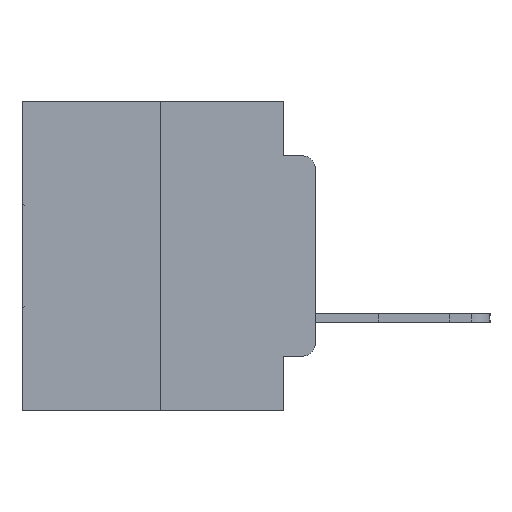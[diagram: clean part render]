
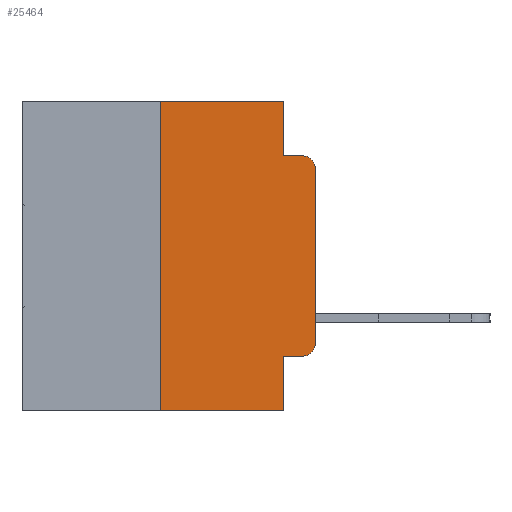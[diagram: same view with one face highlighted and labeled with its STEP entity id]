
A CAD part, left-side view. The second image highlights one B-rep face of the part: STEP entity #25464.
In plain terms, the highlighted planar face has unit normal (-1, 0, 0).
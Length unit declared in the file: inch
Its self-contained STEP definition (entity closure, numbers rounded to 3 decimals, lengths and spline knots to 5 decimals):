
#554 = AXIS2_PLACEMENT_3D ( 'NONE', #18493, #17868, #17990 ) ;
#778 = CARTESIAN_POINT ( 'NONE',  ( 0., 0., -0.1085 ) ) ;
#1525 = EDGE_CURVE ( 'NONE', #25585, #26327, #14648, .T. ) ;
#2395 = ORIENTED_EDGE ( 'NONE', *, *, #7699, .F. ) ;
#3117 = EDGE_CURVE ( 'NONE', #27925, #25585, #3892, .T. ) ;
#3740 = LINE ( 'NONE', #4854, #8344 ) ;
#3865 = DIRECTION ( 'NONE',  ( 0., 0., -1. ) ) ;
#3892 = LINE ( 'NONE', #23694, #26974 ) ;
#4602 = CARTESIAN_POINT ( 'NONE',  ( 0., 0.051, 0. ) ) ;
#4655 = LINE ( 'NONE', #24834, #6081 ) ;
#4662 = EDGE_CURVE ( 'NONE', #27925, #23006, #21340, .T. ) ;
#4854 = CARTESIAN_POINT ( 'NONE',  ( 0., 0.051, -0.0885 ) ) ;
#5065 = VECTOR ( 'NONE', #11693, 39.37008 ) ;
#5301 = CARTESIAN_POINT ( 'NONE',  ( 0., 0.02, -0.0885 ) ) ;
#5423 = ORIENTED_EDGE ( 'NONE', *, *, #21184, .T. ) ;
#6081 = VECTOR ( 'NONE', #16053, 39.37008 ) ;
#6410 = EDGE_CURVE ( 'NONE', #25180, #23006, #28482, .T. ) ;
#7229 = CARTESIAN_POINT ( 'NONE',  ( 0., 0.051, 0. ) ) ;
#7239 = VERTEX_POINT ( 'NONE', #778 ) ;
#7511 = ORIENTED_EDGE ( 'NONE', *, *, #3117, .T. ) ;
#7691 = VECTOR ( 'NONE', #21485, 39.37008 ) ;
#7699 = EDGE_CURVE ( 'NONE', #25180, #12014, #11096, .T. ) ;
#8344 = VECTOR ( 'NONE', #20522, 39.37008 ) ;
#8591 = ORIENTED_EDGE ( 'NONE', *, *, #1525, .T. ) ;
#8647 = CARTESIAN_POINT ( 'NONE',  ( 0., 0.051, -0.5 ) ) ;
#9223 = EDGE_CURVE ( 'NONE', #25778, #20051, #13744, .T. ) ;
#9306 = CARTESIAN_POINT ( 'NONE',  ( 0., 0.473, 0. ) ) ;
#9703 = ORIENTED_EDGE ( 'NONE', *, *, #10740, .F. ) ;
#10339 = DIRECTION ( 'NONE',  ( 0., -1., 0. ) ) ;
#10424 = VECTOR ( 'NONE', #22671, 39.37008 ) ;
#10740 = EDGE_CURVE ( 'NONE', #20051, #24617, #3740, .T. ) ;
#10778 = VECTOR ( 'NONE', #24405, 39.37008 ) ;
#11096 = LINE ( 'NONE', #18317, #5065 ) ;
#11348 = DIRECTION ( 'NONE',  ( 0., 0., -1. ) ) ;
#11401 = DIRECTION ( 'NONE',  ( -1., 0., 0. ) ) ;
#11693 = DIRECTION ( 'NONE',  ( 0., 0., 1. ) ) ;
#12014 = VERTEX_POINT ( 'NONE', #28065 ) ;
#12243 = CARTESIAN_POINT ( 'NONE',  ( 0., 0.051, -0.0885 ) ) ;
#12631 = CIRCLE ( 'NONE', #14117, 0.02 ) ;
#12891 = PLANE ( 'NONE',  #17390 ) ;
#13077 = ORIENTED_EDGE ( 'NONE', *, *, #18103, .F. ) ;
#13744 = LINE ( 'NONE', #21589, #7691 ) ;
#13746 = CARTESIAN_POINT ( 'NONE',  ( 0., 0., -0.3915 ) ) ;
#14117 = AXIS2_PLACEMENT_3D ( 'NONE', #24721, #11401, #26929 ) ;
#14648 = CIRCLE ( 'NONE', #554, 0.02 ) ;
#15046 = LINE ( 'NONE', #9306, #10424 ) ;
#15090 = CARTESIAN_POINT ( 'NONE',  ( 0., 0.473, 0. ) ) ;
#15502 = VECTOR ( 'NONE', #11348, 39.37008 ) ;
#15559 = CARTESIAN_POINT ( 'NONE',  ( 0., 0.02, -0.4115 ) ) ;
#16053 = DIRECTION ( 'NONE',  ( 0., 0., 1. ) ) ;
#16737 = ORIENTED_EDGE ( 'NONE', *, *, #16756, .T. ) ;
#16756 = EDGE_CURVE ( 'NONE', #7239, #24617, #12631, .T. ) ;
#17208 = ORIENTED_EDGE ( 'NONE', *, *, #9223, .F. ) ;
#17357 = DIRECTION ( 'NONE',  ( 1., 0., 0. ) ) ;
#17390 = AXIS2_PLACEMENT_3D ( 'NONE', #15090, #17357, #3865 ) ;
#17868 = DIRECTION ( 'NONE',  ( -1., 0., 0. ) ) ;
#17990 = DIRECTION ( 'NONE',  ( 0., 0., -1. ) ) ;
#18103 = EDGE_CURVE ( 'NONE', #12014, #25778, #15046, .T. ) ;
#18317 = CARTESIAN_POINT ( 'NONE',  ( 0., 0.25, 0. ) ) ;
#18493 = CARTESIAN_POINT ( 'NONE',  ( 0., 0.02, -0.3915 ) ) ;
#18513 = CARTESIAN_POINT ( 'NONE',  ( 0., 0.25, -0.5 ) ) ;
#19915 = CARTESIAN_POINT ( 'NONE',  ( 0., 0.473, -0.5 ) ) ;
#20051 = VERTEX_POINT ( 'NONE', #12243 ) ;
#20522 = DIRECTION ( 'NONE',  ( 0., -1., 0. ) ) ;
#21152 = FACE_OUTER_BOUND ( 'NONE', #21882, .T. ) ;
#21184 = EDGE_CURVE ( 'NONE', #26327, #7239, #4655, .T. ) ;
#21340 = LINE ( 'NONE', #4602, #15502 ) ;
#21485 = DIRECTION ( 'NONE',  ( 0., 0., -1. ) ) ;
#21589 = CARTESIAN_POINT ( 'NONE',  ( 0., 0.051, 0. ) ) ;
#21754 = ORIENTED_EDGE ( 'NONE', *, *, #6410, .T. ) ;
#21882 = EDGE_LOOP ( 'NONE', ( #5423, #16737, #9703, #17208, #13077, #2395, #21754, #23506, #7511, #8591 ) ) ;
#22671 = DIRECTION ( 'NONE',  ( 0., -1., 0. ) ) ;
#23006 = VERTEX_POINT ( 'NONE', #8647 ) ;
#23506 = ORIENTED_EDGE ( 'NONE', *, *, #4662, .F. ) ;
#23694 = CARTESIAN_POINT ( 'NONE',  ( 0., 0.051, -0.4115 ) ) ;
#24405 = DIRECTION ( 'NONE',  ( 0., -1., 0. ) ) ;
#24617 = VERTEX_POINT ( 'NONE', #5301 ) ;
#24721 = CARTESIAN_POINT ( 'NONE',  ( 0., 0.02, -0.1085 ) ) ;
#24834 = CARTESIAN_POINT ( 'NONE',  ( 0., 0., 0. ) ) ;
#25180 = VERTEX_POINT ( 'NONE', #18513 ) ;
#25464 = ADVANCED_FACE ( 'NONE', ( #21152 ), #12891, .F. ) ;
#25585 = VERTEX_POINT ( 'NONE', #15559 ) ;
#25778 = VERTEX_POINT ( 'NONE', #7229 ) ;
#25864 = CARTESIAN_POINT ( 'NONE',  ( 0., 0.051, -0.4115 ) ) ;
#26327 = VERTEX_POINT ( 'NONE', #13746 ) ;
#26929 = DIRECTION ( 'NONE',  ( 0., 0., -1. ) ) ;
#26974 = VECTOR ( 'NONE', #10339, 39.37008 ) ;
#27925 = VERTEX_POINT ( 'NONE', #25864 ) ;
#28065 = CARTESIAN_POINT ( 'NONE',  ( 0., 0.25, 0. ) ) ;
#28482 = LINE ( 'NONE', #19915, #10778 ) ;
